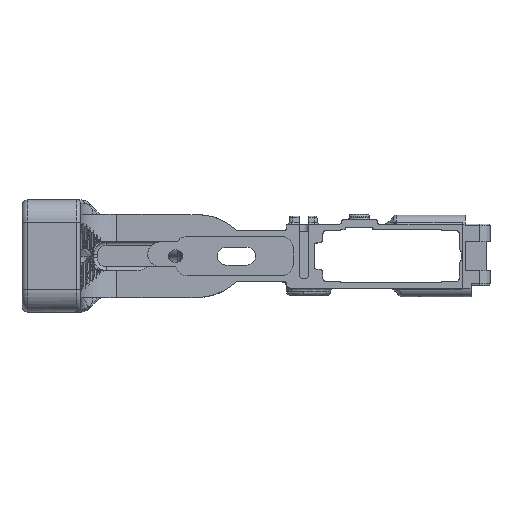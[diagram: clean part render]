
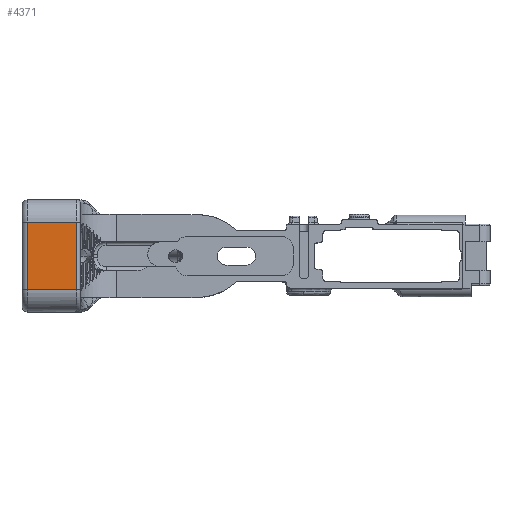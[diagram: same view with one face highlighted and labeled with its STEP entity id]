
A CAD part, top view. The second image highlights one B-rep face of the part: STEP entity #4371.
In plain terms, the highlighted planar face has unit normal (0, 0, 1).
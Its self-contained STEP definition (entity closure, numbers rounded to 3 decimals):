
#1927 = VECTOR ( 'NONE', #30996, 1000. ) ;
#3096 = ORIENTED_EDGE ( 'NONE', *, *, #26245, .T. ) ;
#4371 = ADVANCED_FACE ( 'NONE', ( #53764 ), #8702, .T. ) ;
#6924 = ORIENTED_EDGE ( 'NONE', *, *, #23771, .T. ) ;
#7688 = LINE ( 'NONE', #34631, #39888 ) ;
#8702 = PLANE ( 'NONE',  #45141 ) ;
#13790 = VERTEX_POINT ( 'NONE', #24091 ) ;
#14318 = DIRECTION ( 'NONE',  ( -1., 0., 0. ) ) ;
#14360 = CARTESIAN_POINT ( 'NONE',  ( -78.86, -34.921, 52.476 ) ) ;
#14503 = EDGE_CURVE ( 'NONE', #18856, #36824, #53161, .T. ) ;
#18856 = VERTEX_POINT ( 'NONE', #56684 ) ;
#21033 = VECTOR ( 'NONE', #44992, 1000. ) ;
#22769 = CARTESIAN_POINT ( 'NONE',  ( -89.794, -44.921, 52.476 ) ) ;
#22886 = DIRECTION ( 'NONE',  ( -1., 0., 0. ) ) ;
#22977 = CARTESIAN_POINT ( 'NONE',  ( -78.86, -4.921, 52.476 ) ) ;
#23727 = ORIENTED_EDGE ( 'NONE', *, *, #14503, .F. ) ;
#23771 = EDGE_CURVE ( 'NONE', #37577, #13790, #34310, .T. ) ;
#24091 = CARTESIAN_POINT ( 'NONE',  ( -89.794, -4.921, 52.476 ) ) ;
#26245 = EDGE_CURVE ( 'NONE', #18856, #37577, #7688, .T. ) ;
#30996 = DIRECTION ( 'NONE',  ( 0., -1., 0. ) ) ;
#31911 = EDGE_CURVE ( 'NONE', #13790, #36824, #35503, .T. ) ;
#34310 = LINE ( 'NONE', #22977, #54802 ) ;
#34443 = DIRECTION ( 'NONE',  ( 0., 1., 0. ) ) ;
#34631 = CARTESIAN_POINT ( 'NONE',  ( -67.834, -4.921, 52.476 ) ) ;
#35012 = CARTESIAN_POINT ( 'NONE',  ( -89.794, -34.921, 52.476 ) ) ;
#35503 = LINE ( 'NONE', #22769, #1927 ) ;
#36824 = VERTEX_POINT ( 'NONE', #35012 ) ;
#37577 = VERTEX_POINT ( 'NONE', #47884 ) ;
#39888 = VECTOR ( 'NONE', #34443, 1000. ) ;
#44676 = CARTESIAN_POINT ( 'NONE',  ( -78.86, -44.921, 52.476 ) ) ;
#44992 = DIRECTION ( 'NONE',  ( -1., 0., 0. ) ) ;
#45141 = AXIS2_PLACEMENT_3D ( 'NONE', #44676, #49069, #22886 ) ;
#47884 = CARTESIAN_POINT ( 'NONE',  ( -67.834, -4.921, 52.476 ) ) ;
#49069 = DIRECTION ( 'NONE',  ( 0., 0., 1. ) ) ;
#49116 = EDGE_LOOP ( 'NONE', ( #6924, #50035, #23727, #3096 ) ) ;
#50035 = ORIENTED_EDGE ( 'NONE', *, *, #31911, .T. ) ;
#53161 = LINE ( 'NONE', #14360, #21033 ) ;
#53764 = FACE_OUTER_BOUND ( 'NONE', #49116, .T. ) ;
#54802 = VECTOR ( 'NONE', #14318, 1000. ) ;
#56684 = CARTESIAN_POINT ( 'NONE',  ( -67.834, -34.921, 52.476 ) ) ;
